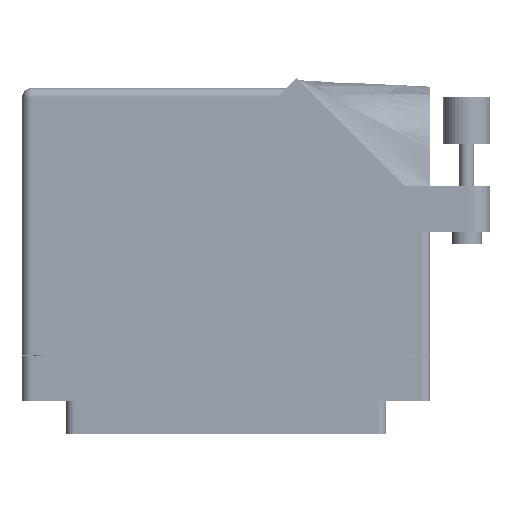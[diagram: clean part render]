
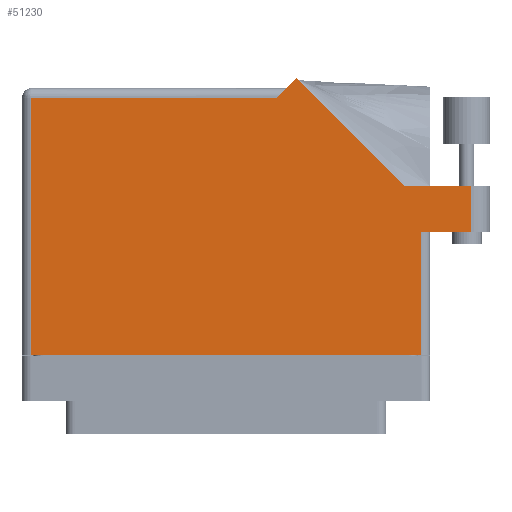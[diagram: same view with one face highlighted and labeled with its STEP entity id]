
A CAD part, front view. The second image highlights one B-rep face of the part: STEP entity #51230.
In plain terms, the highlighted face is planar.
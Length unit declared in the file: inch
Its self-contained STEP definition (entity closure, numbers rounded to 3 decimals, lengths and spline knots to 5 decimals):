
#523 = LINE ( 'NONE', #7109, #59893 ) ;
#1772 = VECTOR ( 'NONE', #31299, 39.37008 ) ;
#1788 = VECTOR ( 'NONE', #13991, 39.37008 ) ;
#2108 = CARTESIAN_POINT ( 'NONE',  ( -1.359, -0.1, 0.617 ) ) ;
#2666 = VECTOR ( 'NONE', #68839, 39.37008 ) ;
#2815 = CARTESIAN_POINT ( 'NONE',  ( -1.297, 1.613, 0.617 ) ) ;
#3072 = DIRECTION ( 'NONE',  ( -0.707, 0.707, 0. ) ) ;
#6394 = DIRECTION ( 'NONE',  ( 0., 1., 0. ) ) ;
#6629 = CARTESIAN_POINT ( 'NONE',  ( 1.19342, 1.022, 0.617 ) ) ;
#6683 = VERTEX_POINT ( 'NONE', #42718 ) ;
#7109 = CARTESIAN_POINT ( 'NONE',  ( 0.399, 1.675, 0.617 ) ) ;
#7648 = VERTEX_POINT ( 'NONE', #50690 ) ;
#7848 = AXIS2_PLACEMENT_3D ( 'NONE', #26631, #65196, #42893 ) ;
#9490 = EDGE_CURVE ( 'NONE', #44619, #22190, #29144, .T. ) ;
#10299 = EDGE_CURVE ( 'NONE', #22190, #38225, #17166, .T. ) ;
#12159 = CARTESIAN_POINT ( 'NONE',  ( 0.46971, 1.74571, 0.617 ) ) ;
#13726 = LINE ( 'NONE', #58307, #1772 ) ;
#13991 = DIRECTION ( 'NONE',  ( 1., 0., 0. ) ) ;
#16054 = VERTEX_POINT ( 'NONE', #2815 ) ;
#16848 = VECTOR ( 'NONE', #3072, 39.37008 ) ;
#17166 = LINE ( 'NONE', #63354, #2666 ) ;
#19723 = CARTESIAN_POINT ( 'NONE',  ( 1.359, 0.715, 0.617 ) ) ;
#19791 = EDGE_CURVE ( 'NONE', #16054, #28797, #68419, .T. ) ;
#20425 = DIRECTION ( 'NONE',  ( 1., 0., 0. ) ) ;
#21414 = LINE ( 'NONE', #2108, #1788 ) ;
#21892 = EDGE_CURVE ( 'NONE', #6683, #44619, #65218, .T. ) ;
#22190 = VERTEX_POINT ( 'NONE', #70071 ) ;
#22796 = EDGE_LOOP ( 'NONE', ( #23609, #36797, #57472, #41474, #42540, #30656, #65842, #26906, #51798 ) ) ;
#23089 = CARTESIAN_POINT ( 'NONE',  ( 1.297, 0.715, 0.617 ) ) ;
#23609 = ORIENTED_EDGE ( 'NONE', *, *, #21892, .T. ) ;
#26177 = CARTESIAN_POINT ( 'NONE',  ( 1.634, 1.022, 0.617 ) ) ;
#26631 = CARTESIAN_POINT ( 'NONE',  ( -1.359, 1.675, 0.617 ) ) ;
#26906 = ORIENTED_EDGE ( 'NONE', *, *, #32525, .T. ) ;
#27109 = DIRECTION ( 'NONE',  ( 0., 1., 0. ) ) ;
#27945 = CARTESIAN_POINT ( 'NONE',  ( -1.297, -0.1, 0.617 ) ) ;
#28797 = VERTEX_POINT ( 'NONE', #27945 ) ;
#29144 = LINE ( 'NONE', #26177, #59617 ) ;
#30656 = ORIENTED_EDGE ( 'NONE', *, *, #50162, .T. ) ;
#31299 = DIRECTION ( 'NONE',  ( -1., 0., 0. ) ) ;
#32251 = PLANE ( 'NONE',  #7848 ) ;
#32525 = EDGE_CURVE ( 'NONE', #28797, #7648, #21414, .T. ) ;
#34439 = VECTOR ( 'NONE', #56046, 39.37008 ) ;
#34885 = EDGE_CURVE ( 'NONE', #47959, #47860, #523, .T. ) ;
#36339 = VECTOR ( 'NONE', #6394, 39.37008 ) ;
#36797 = ORIENTED_EDGE ( 'NONE', *, *, #9490, .T. ) ;
#38225 = VERTEX_POINT ( 'NONE', #6629 ) ;
#41467 = VECTOR ( 'NONE', #20425, 39.37008 ) ;
#41474 = ORIENTED_EDGE ( 'NONE', *, *, #45768, .T. ) ;
#42423 = CARTESIAN_POINT ( 'NONE',  ( 1.634, 0.715, 0.617 ) ) ;
#42540 = ORIENTED_EDGE ( 'NONE', *, *, #34885, .T. ) ;
#42718 = CARTESIAN_POINT ( 'NONE',  ( 1.297, 0.715, 0.617 ) ) ;
#42893 = DIRECTION ( 'NONE',  ( -1., 0., 0. ) ) ;
#44619 = VERTEX_POINT ( 'NONE', #42423 ) ;
#45084 = CARTESIAN_POINT ( 'NONE',  ( -1.297, -0.1, 0.617 ) ) ;
#45700 = EDGE_CURVE ( 'NONE', #7648, #6683, #67724, .T. ) ;
#45768 = EDGE_CURVE ( 'NONE', #38225, #47959, #51549, .T. ) ;
#47860 = VERTEX_POINT ( 'NONE', #50898 ) ;
#47959 = VERTEX_POINT ( 'NONE', #12159 ) ;
#49810 = DIRECTION ( 'NONE',  ( -0.707, -0.707, 0. ) ) ;
#49994 = FACE_OUTER_BOUND ( 'NONE', #22796, .T. ) ;
#50162 = EDGE_CURVE ( 'NONE', #47860, #16054, #13726, .T. ) ;
#50690 = CARTESIAN_POINT ( 'NONE',  ( 1.297, -0.1, 0.617 ) ) ;
#50898 = CARTESIAN_POINT ( 'NONE',  ( 0.337, 1.613, 0.617 ) ) ;
#51230 = ADVANCED_FACE ( 'NONE', ( #49994 ), #32251, .F. ) ;
#51549 = LINE ( 'NONE', #66921, #16848 ) ;
#51798 = ORIENTED_EDGE ( 'NONE', *, *, #45700, .T. ) ;
#56046 = DIRECTION ( 'NONE',  ( 0., -1., 0. ) ) ;
#57472 = ORIENTED_EDGE ( 'NONE', *, *, #10299, .T. ) ;
#58307 = CARTESIAN_POINT ( 'NONE',  ( -1.359, 1.613, 0.617 ) ) ;
#59617 = VECTOR ( 'NONE', #27109, 39.37008 ) ;
#59893 = VECTOR ( 'NONE', #49810, 39.37008 ) ;
#63354 = CARTESIAN_POINT ( 'NONE',  ( 1.759, 1.022, 0.617 ) ) ;
#65196 = DIRECTION ( 'NONE',  ( 0., 0., -1. ) ) ;
#65218 = LINE ( 'NONE', #19723, #41467 ) ;
#65842 = ORIENTED_EDGE ( 'NONE', *, *, #19791, .T. ) ;
#66921 = CARTESIAN_POINT ( 'NONE',  ( 1.19342, 1.022, 0.617 ) ) ;
#67724 = LINE ( 'NONE', #23089, #36339 ) ;
#68419 = LINE ( 'NONE', #45084, #34439 ) ;
#68839 = DIRECTION ( 'NONE',  ( -1., 0., 0. ) ) ;
#70071 = CARTESIAN_POINT ( 'NONE',  ( 1.634, 1.022, 0.617 ) ) ;
